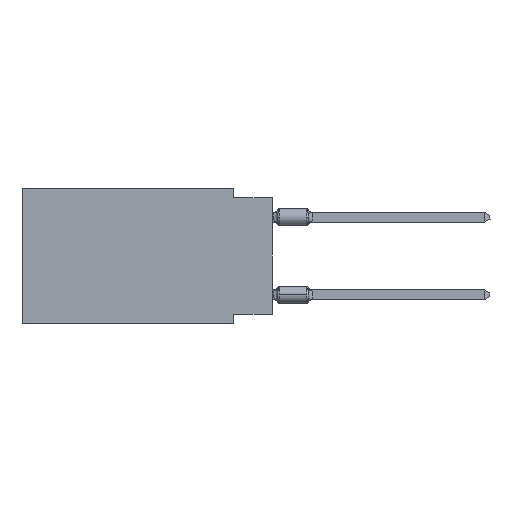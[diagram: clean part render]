
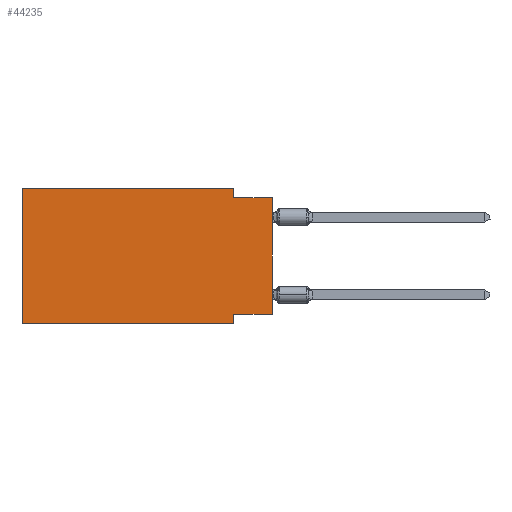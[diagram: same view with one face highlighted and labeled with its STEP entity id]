
A CAD part, left-side view. The second image highlights one B-rep face of the part: STEP entity #44235.
In plain terms, the highlighted planar face has unit normal (-1, 0, 0).
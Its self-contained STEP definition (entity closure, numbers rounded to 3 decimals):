
#373 = VERTEX_POINT ( 'NONE', #55060 ) ;
#726 = VERTEX_POINT ( 'NONE', #45587 ) ;
#904 = DIRECTION ( 'NONE',  ( 0., 0., -1. ) ) ;
#2592 = ORIENTED_EDGE ( 'NONE', *, *, #41447, .F. ) ;
#4347 = CARTESIAN_POINT ( 'NONE',  ( 0., 0., -8.255 ) ) ;
#5421 = CARTESIAN_POINT ( 'NONE',  ( 0., 2.54, -0.635 ) ) ;
#5440 = CARTESIAN_POINT ( 'NONE',  ( 0., 16.383, 0. ) ) ;
#6768 = CARTESIAN_POINT ( 'NONE',  ( 0., 2.54, -8.89 ) ) ;
#7570 = VERTEX_POINT ( 'NONE', #49660 ) ;
#8865 = CARTESIAN_POINT ( 'NONE',  ( 0., 0., -8.255 ) ) ;
#9420 = LINE ( 'NONE', #50024, #32964 ) ;
#9561 = VECTOR ( 'NONE', #35507, 1000. ) ;
#10085 = EDGE_CURVE ( 'NONE', #34240, #50677, #53710, .T. ) ;
#10900 = DIRECTION ( 'NONE',  ( 0., -1., 0. ) ) ;
#11368 = EDGE_CURVE ( 'NONE', #51475, #726, #48449, .T. ) ;
#11999 = LINE ( 'NONE', #49867, #32531 ) ;
#13310 = CARTESIAN_POINT ( 'NONE',  ( 0., 0., -0.635 ) ) ;
#13529 = EDGE_CURVE ( 'NONE', #373, #43978, #9420, .T. ) ;
#13712 = EDGE_CURVE ( 'NONE', #51475, #43978, #33933, .T. ) ;
#14632 = LINE ( 'NONE', #51586, #33432 ) ;
#18276 = DIRECTION ( 'NONE',  ( 0., 1., 0. ) ) ;
#18482 = VECTOR ( 'NONE', #10900, 1000. ) ;
#19075 = ORIENTED_EDGE ( 'NONE', *, *, #11368, .F. ) ;
#20666 = EDGE_CURVE ( 'NONE', #7570, #49520, #11999, .T. ) ;
#23464 = ORIENTED_EDGE ( 'NONE', *, *, #13712, .T. ) ;
#24163 = VECTOR ( 'NONE', #35608, 1000. ) ;
#26775 = ORIENTED_EDGE ( 'NONE', *, *, #34260, .F. ) ;
#26799 = CARTESIAN_POINT ( 'NONE',  ( 0., 16.383, -8.89 ) ) ;
#27355 = LINE ( 'NONE', #4347, #56059 ) ;
#27812 = ORIENTED_EDGE ( 'NONE', *, *, #47776, .F. ) ;
#27936 = ORIENTED_EDGE ( 'NONE', *, *, #10085, .T. ) ;
#28601 = ORIENTED_EDGE ( 'NONE', *, *, #13529, .F. ) ;
#30185 = CARTESIAN_POINT ( 'NONE',  ( 0., 0., -0.635 ) ) ;
#30776 = LINE ( 'NONE', #30185, #24163 ) ;
#32397 = FACE_OUTER_BOUND ( 'NONE', #37202, .T. ) ;
#32531 = VECTOR ( 'NONE', #34724, 1000. ) ;
#32964 = VECTOR ( 'NONE', #41529, 1000. ) ;
#33432 = VECTOR ( 'NONE', #37934, 1000. ) ;
#33933 = LINE ( 'NONE', #55799, #18482 ) ;
#34240 = VERTEX_POINT ( 'NONE', #8865 ) ;
#34260 = EDGE_CURVE ( 'NONE', #726, #7570, #14632, .T. ) ;
#34724 = DIRECTION ( 'NONE',  ( 0., 0., -1. ) ) ;
#35507 = DIRECTION ( 'NONE',  ( 0., 0., 1. ) ) ;
#35608 = DIRECTION ( 'NONE',  ( 0., -1., 0. ) ) ;
#37202 = EDGE_LOOP ( 'NONE', ( #27936, #27812, #40118, #26775, #19075, #23464, #28601, #2592 ) ) ;
#37934 = DIRECTION ( 'NONE',  ( 0., -1., 0. ) ) ;
#40118 = ORIENTED_EDGE ( 'NONE', *, *, #20666, .F. ) ;
#41447 = EDGE_CURVE ( 'NONE', #34240, #373, #27355, .T. ) ;
#41529 = DIRECTION ( 'NONE',  ( 0., 0., -1. ) ) ;
#43893 = CARTESIAN_POINT ( 'NONE',  ( 0., 16.383, 0. ) ) ;
#43978 = VERTEX_POINT ( 'NONE', #6768 ) ;
#44235 = ADVANCED_FACE ( 'NONE', ( #32397 ), #51495, .F. ) ;
#44611 = CARTESIAN_POINT ( 'NONE',  ( 0., 0., 0. ) ) ;
#45587 = CARTESIAN_POINT ( 'NONE',  ( 0., 16.383, 0. ) ) ;
#47776 = EDGE_CURVE ( 'NONE', #49520, #50677, #30776, .T. ) ;
#48449 = LINE ( 'NONE', #43893, #50208 ) ;
#49520 = VERTEX_POINT ( 'NONE', #5421 ) ;
#49660 = CARTESIAN_POINT ( 'NONE',  ( 0., 2.54, 0. ) ) ;
#49867 = CARTESIAN_POINT ( 'NONE',  ( 0., 2.54, 0. ) ) ;
#50024 = CARTESIAN_POINT ( 'NONE',  ( 0., 2.54, -8.89 ) ) ;
#50208 = VECTOR ( 'NONE', #53296, 1000. ) ;
#50677 = VERTEX_POINT ( 'NONE', #13310 ) ;
#51416 = AXIS2_PLACEMENT_3D ( 'NONE', #5440, #56645, #904 ) ;
#51475 = VERTEX_POINT ( 'NONE', #26799 ) ;
#51495 = PLANE ( 'NONE',  #51416 ) ;
#51586 = CARTESIAN_POINT ( 'NONE',  ( 0., 16.383, 0. ) ) ;
#53296 = DIRECTION ( 'NONE',  ( 0., 0., 1. ) ) ;
#53710 = LINE ( 'NONE', #44611, #9561 ) ;
#55060 = CARTESIAN_POINT ( 'NONE',  ( 0., 2.54, -8.255 ) ) ;
#55799 = CARTESIAN_POINT ( 'NONE',  ( 0., 16.383, -8.89 ) ) ;
#56059 = VECTOR ( 'NONE', #18276, 1000. ) ;
#56645 = DIRECTION ( 'NONE',  ( 1., 0., 0. ) ) ;
